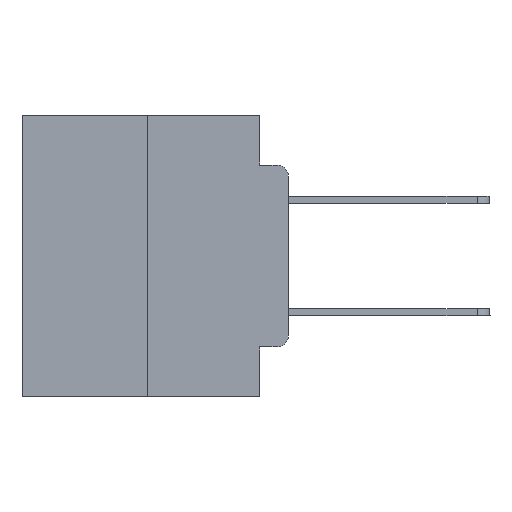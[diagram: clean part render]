
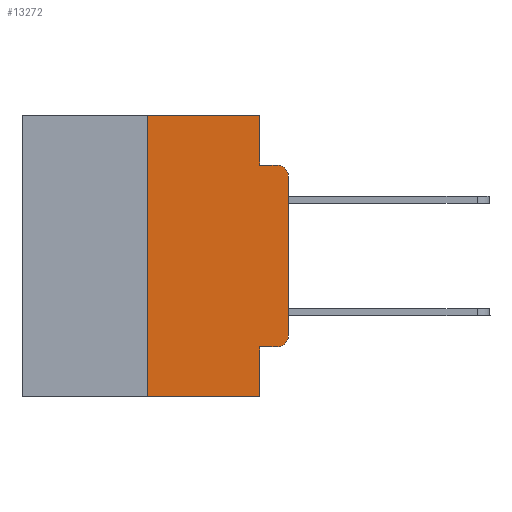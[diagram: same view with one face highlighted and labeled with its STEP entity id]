
A CAD part, left-side view. The second image highlights one B-rep face of the part: STEP entity #13272.
In plain terms, the highlighted planar face has unit normal (-1, 0, 0).
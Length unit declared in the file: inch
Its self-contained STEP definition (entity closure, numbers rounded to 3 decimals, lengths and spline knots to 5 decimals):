
#443 = DIRECTION ( 'NONE',  ( -1., 0., 0. ) ) ;
#1004 = VECTOR ( 'NONE', #19631, 39.37008 ) ;
#1340 = VECTOR ( 'NONE', #19184, 39.37008 ) ;
#1469 = ORIENTED_EDGE ( 'NONE', *, *, #7376, .T. ) ;
#1470 = CARTESIAN_POINT ( 'NONE',  ( 0., 0., -0.1085 ) ) ;
#1642 = LINE ( 'NONE', #11744, #21143 ) ;
#1694 = LINE ( 'NONE', #3976, #7384 ) ;
#1939 = VERTEX_POINT ( 'NONE', #25843 ) ;
#2223 = VERTEX_POINT ( 'NONE', #6840 ) ;
#2659 = EDGE_CURVE ( 'NONE', #9449, #16127, #18768, .T. ) ;
#2760 = VERTEX_POINT ( 'NONE', #20946 ) ;
#2784 = CARTESIAN_POINT ( 'NONE',  ( 0., 0.473, -0.5 ) ) ;
#2870 = CARTESIAN_POINT ( 'NONE',  ( 0., 0.02, -0.1085 ) ) ;
#2910 = VECTOR ( 'NONE', #19487, 39.37008 ) ;
#3021 = CARTESIAN_POINT ( 'NONE',  ( 0., 0.473, 0. ) ) ;
#3126 = CIRCLE ( 'NONE', #4007, 0.02 ) ;
#3215 = CARTESIAN_POINT ( 'NONE',  ( 0., 0.051, -0.0885 ) ) ;
#3231 = ORIENTED_EDGE ( 'NONE', *, *, #26228, .F. ) ;
#3568 = DIRECTION ( 'NONE',  ( 0., 0., -1. ) ) ;
#3828 = DIRECTION ( 'NONE',  ( 1., 0., 0. ) ) ;
#3976 = CARTESIAN_POINT ( 'NONE',  ( 0., 0.25, 0. ) ) ;
#4007 = AXIS2_PLACEMENT_3D ( 'NONE', #2870, #19294, #9083 ) ;
#4100 = PLANE ( 'NONE',  #15609 ) ;
#4176 = VERTEX_POINT ( 'NONE', #21127 ) ;
#4186 = EDGE_CURVE ( 'NONE', #16346, #16127, #9134, .T. ) ;
#4648 = CARTESIAN_POINT ( 'NONE',  ( 0., 0.051, 0. ) ) ;
#5249 = VERTEX_POINT ( 'NONE', #1470 ) ;
#5472 = VECTOR ( 'NONE', #19458, 39.37008 ) ;
#5944 = EDGE_CURVE ( 'NONE', #2760, #4176, #18915, .T. ) ;
#6840 = CARTESIAN_POINT ( 'NONE',  ( 0., 0.02, -0.4115 ) ) ;
#6928 = CARTESIAN_POINT ( 'NONE',  ( 0., 0.02, -0.3915 ) ) ;
#7376 = EDGE_CURVE ( 'NONE', #1939, #5249, #17429, .T. ) ;
#7384 = VECTOR ( 'NONE', #8030, 39.37008 ) ;
#8030 = DIRECTION ( 'NONE',  ( 0., 0., 1. ) ) ;
#8680 = DIRECTION ( 'NONE',  ( 0., 0., -1. ) ) ;
#8798 = EDGE_CURVE ( 'NONE', #4176, #19997, #1642, .T. ) ;
#9083 = DIRECTION ( 'NONE',  ( 0., 0., -1. ) ) ;
#9099 = EDGE_CURVE ( 'NONE', #9449, #2223, #11418, .T. ) ;
#9134 = LINE ( 'NONE', #2784, #2910 ) ;
#9449 = VERTEX_POINT ( 'NONE', #12875 ) ;
#9809 = EDGE_CURVE ( 'NONE', #2223, #1939, #14595, .T. ) ;
#9928 = CARTESIAN_POINT ( 'NONE',  ( 0., 0.051, -0.5 ) ) ;
#11418 = LINE ( 'NONE', #25972, #1004 ) ;
#11744 = CARTESIAN_POINT ( 'NONE',  ( 0., 0.051, 0. ) ) ;
#12004 = DIRECTION ( 'NONE',  ( 0., 0., -1. ) ) ;
#12875 = CARTESIAN_POINT ( 'NONE',  ( 0., 0.051, -0.4115 ) ) ;
#12879 = AXIS2_PLACEMENT_3D ( 'NONE', #6928, #443, #8680 ) ;
#12989 = DIRECTION ( 'NONE',  ( 0., 0., -1. ) ) ;
#13272 = ADVANCED_FACE ( 'NONE', ( #22300 ), #4100, .F. ) ;
#13424 = VERTEX_POINT ( 'NONE', #24573 ) ;
#13599 = LINE ( 'NONE', #3215, #14208 ) ;
#13671 = ORIENTED_EDGE ( 'NONE', *, *, #2659, .F. ) ;
#13684 = EDGE_CURVE ( 'NONE', #5249, #13424, #3126, .T. ) ;
#13815 = CARTESIAN_POINT ( 'NONE',  ( 0., 0.473, 0. ) ) ;
#14208 = VECTOR ( 'NONE', #15351, 39.37008 ) ;
#14595 = CIRCLE ( 'NONE', #12879, 0.02 ) ;
#15351 = DIRECTION ( 'NONE',  ( 0., -1., 0. ) ) ;
#15609 = AXIS2_PLACEMENT_3D ( 'NONE', #13815, #3828, #3568 ) ;
#16127 = VERTEX_POINT ( 'NONE', #9928 ) ;
#16346 = VERTEX_POINT ( 'NONE', #20287 ) ;
#16720 = CARTESIAN_POINT ( 'NONE',  ( 0., 0.051, -0.0885 ) ) ;
#16740 = ORIENTED_EDGE ( 'NONE', *, *, #13684, .T. ) ;
#16872 = ORIENTED_EDGE ( 'NONE', *, *, #8798, .F. ) ;
#16903 = VECTOR ( 'NONE', #12989, 39.37008 ) ;
#16957 = EDGE_LOOP ( 'NONE', ( #1469, #16740, #25107, #16872, #22892, #3231, #24695, #13671, #17506, #25836 ) ) ;
#17429 = LINE ( 'NONE', #25527, #5472 ) ;
#17506 = ORIENTED_EDGE ( 'NONE', *, *, #9099, .T. ) ;
#18768 = LINE ( 'NONE', #4648, #16903 ) ;
#18915 = LINE ( 'NONE', #3021, #1340 ) ;
#19184 = DIRECTION ( 'NONE',  ( 0., -1., 0. ) ) ;
#19294 = DIRECTION ( 'NONE',  ( -1., 0., 0. ) ) ;
#19458 = DIRECTION ( 'NONE',  ( 0., 0., 1. ) ) ;
#19487 = DIRECTION ( 'NONE',  ( 0., -1., 0. ) ) ;
#19631 = DIRECTION ( 'NONE',  ( 0., -1., 0. ) ) ;
#19997 = VERTEX_POINT ( 'NONE', #16720 ) ;
#20287 = CARTESIAN_POINT ( 'NONE',  ( 0., 0.25, -0.5 ) ) ;
#20946 = CARTESIAN_POINT ( 'NONE',  ( 0., 0.25, 0. ) ) ;
#21127 = CARTESIAN_POINT ( 'NONE',  ( 0., 0.051, 0. ) ) ;
#21143 = VECTOR ( 'NONE', #12004, 39.37008 ) ;
#22083 = EDGE_CURVE ( 'NONE', #19997, #13424, #13599, .T. ) ;
#22300 = FACE_OUTER_BOUND ( 'NONE', #16957, .T. ) ;
#22892 = ORIENTED_EDGE ( 'NONE', *, *, #5944, .F. ) ;
#24573 = CARTESIAN_POINT ( 'NONE',  ( 0., 0.02, -0.0885 ) ) ;
#24695 = ORIENTED_EDGE ( 'NONE', *, *, #4186, .T. ) ;
#25107 = ORIENTED_EDGE ( 'NONE', *, *, #22083, .F. ) ;
#25527 = CARTESIAN_POINT ( 'NONE',  ( 0., 0., 0. ) ) ;
#25836 = ORIENTED_EDGE ( 'NONE', *, *, #9809, .T. ) ;
#25843 = CARTESIAN_POINT ( 'NONE',  ( 0., 0., -0.3915 ) ) ;
#25972 = CARTESIAN_POINT ( 'NONE',  ( 0., 0.051, -0.4115 ) ) ;
#26228 = EDGE_CURVE ( 'NONE', #16346, #2760, #1694, .T. ) ;
